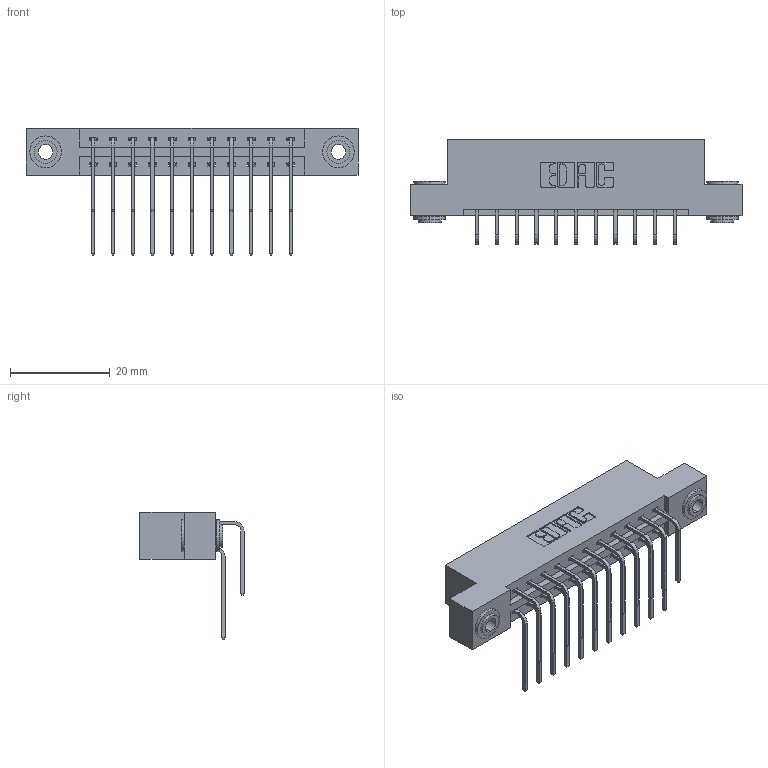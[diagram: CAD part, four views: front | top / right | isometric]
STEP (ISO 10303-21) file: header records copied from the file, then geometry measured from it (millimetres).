
FILE_DESCRIPTION (( 'STEP AP203' ), '1' );
FILE_NAME ('387-022-559-203.STEP', '2018-09-14T06:43:51', ( '' ), ( '' ), 'SwSTEP 2.0', 'SolidWorks 2016', '' );
FILE_SCHEMA (( 'CONFIG_CONTROL_DESIGN' ));
Length unit declared in the file: inch
Products named in the file (5): 387-022-559-203; 337 Part_Flush Mounting Lugs - 0.156 Dia-TH; 345-292-001_558 559 Tail - 1; 345-292-001_559 Tail - 2; 345-250-002_345-250-002-102
Assembly tree (25 placements, depth 2):
  387-022-559-203
    337 Part_Flush Mounting Lugs - 0.156 Dia-TH
    345-292-001_558 559 Tail - 1  x11
    345-292-001_559 Tail - 2  x11
    345-250-002_345-250-002-102  x2
Bounding box: 66.6 x 20.9 x 25.53 mm (x, y, z)
Volume: 6752.4 mm3; surface area: 8194.1 mm2
Topology: 25 solids, 25 shells, 1384 faces, 4061 edges, 2674 vertices
Faces by surface type: plane 960, cylinder 416, cone 8
Entity records: 14972 total; most frequent: CARTESIAN_POINT 2568, ORIENTED_EDGE 2446, DIRECTION 2257, EDGE_CURVE 1223, LINE 1031, VECTOR 1031, VERTEX_POINT 810, AXIS2_PLACEMENT_3D 613
